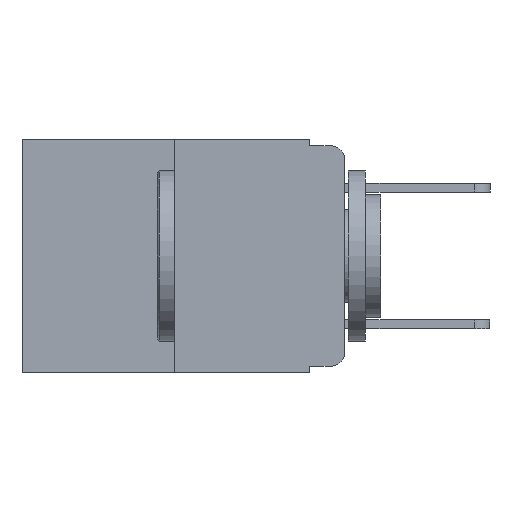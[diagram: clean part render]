
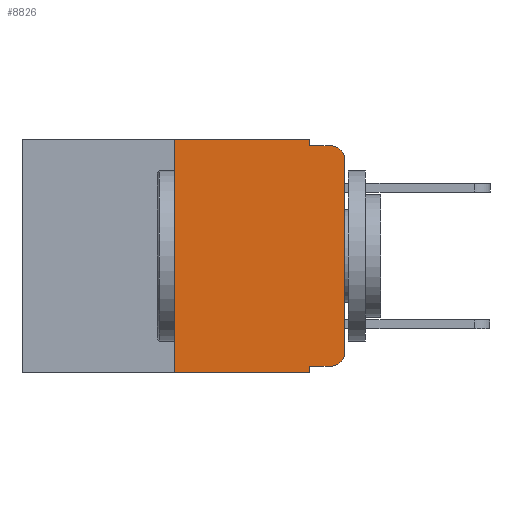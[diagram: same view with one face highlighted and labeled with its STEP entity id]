
A CAD part, left-side view. The second image highlights one B-rep face of the part: STEP entity #8826.
In plain terms, the highlighted planar face has unit normal (-1, 0, 0).
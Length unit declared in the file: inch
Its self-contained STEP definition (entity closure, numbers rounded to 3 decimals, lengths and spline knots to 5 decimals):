
#76 = ORIENTED_EDGE ( 'NONE', *, *, #11005, .F. ) ;
#257 = EDGE_CURVE ( 'NONE', #10354, #1888, #15222, .T. ) ;
#269 = DIRECTION ( 'NONE',  ( 1., 0., 0. ) ) ;
#712 = AXIS2_PLACEMENT_3D ( 'NONE', #13925, #269, #10155 ) ;
#747 = LINE ( 'NONE', #17176, #7976 ) ;
#757 = CARTESIAN_POINT ( 'NONE',  ( 0., 0., -0.313 ) ) ;
#927 = VECTOR ( 'NONE', #12690, 39.37008 ) ;
#973 = VECTOR ( 'NONE', #11604, 39.37008 ) ;
#1206 = EDGE_CURVE ( 'NONE', #1888, #14807, #6623, .T. ) ;
#1469 = LINE ( 'NONE', #15283, #973 ) ;
#1518 = CARTESIAN_POINT ( 'NONE',  ( 0., 0.02, -0.01 ) ) ;
#1888 = VERTEX_POINT ( 'NONE', #11356 ) ;
#2137 = ORIENTED_EDGE ( 'NONE', *, *, #10632, .T. ) ;
#2163 = VECTOR ( 'NONE', #12862, 39.37008 ) ;
#2236 = EDGE_CURVE ( 'NONE', #11568, #10518, #9828, .T. ) ;
#2255 = EDGE_CURVE ( 'NONE', #17080, #9386, #5489, .T. ) ;
#2849 = DIRECTION ( 'NONE',  ( 0., -1., 0. ) ) ;
#3231 = CARTESIAN_POINT ( 'NONE',  ( 0., 0.051, -0.01 ) ) ;
#3321 = EDGE_CURVE ( 'NONE', #9386, #14807, #747, .T. ) ;
#3377 = PLANE ( 'NONE',  #712 ) ;
#3737 = DIRECTION ( 'NONE',  ( 0., -1., 0. ) ) ;
#4075 = ORIENTED_EDGE ( 'NONE', *, *, #2236, .F. ) ;
#4689 = EDGE_CURVE ( 'NONE', #10503, #7376, #1469, .T. ) ;
#4737 = EDGE_CURVE ( 'NONE', #11568, #14059, #14131, .T. ) ;
#5237 = ORIENTED_EDGE ( 'NONE', *, *, #3321, .F. ) ;
#5489 = LINE ( 'NONE', #14955, #8638 ) ;
#5606 = CARTESIAN_POINT ( 'NONE',  ( 0., 0.02, -0.313 ) ) ;
#5688 = AXIS2_PLACEMENT_3D ( 'NONE', #5606, #14610, #6977 ) ;
#6395 = CARTESIAN_POINT ( 'NONE',  ( 0., 0.473, 0. ) ) ;
#6471 = CARTESIAN_POINT ( 'NONE',  ( 0., 0.051, -0.333 ) ) ;
#6623 = CIRCLE ( 'NONE', #15960, 0.02 ) ;
#6977 = DIRECTION ( 'NONE',  ( 0., 0., -1. ) ) ;
#7217 = DIRECTION ( 'NONE',  ( 0., 0., -1. ) ) ;
#7234 = EDGE_CURVE ( 'NONE', #14059, #10354, #10502, .T. ) ;
#7376 = VERTEX_POINT ( 'NONE', #16024 ) ;
#7976 = VECTOR ( 'NONE', #15986, 39.37008 ) ;
#8301 = CARTESIAN_POINT ( 'NONE',  ( 0., 0.051, -0.333 ) ) ;
#8638 = VECTOR ( 'NONE', #12142, 39.37008 ) ;
#8648 = ORIENTED_EDGE ( 'NONE', *, *, #2255, .F. ) ;
#8799 = ORIENTED_EDGE ( 'NONE', *, *, #1206, .T. ) ;
#8826 = ADVANCED_FACE ( 'NONE', ( #9641 ), #3377, .F. ) ;
#9386 = VERTEX_POINT ( 'NONE', #3231 ) ;
#9641 = FACE_OUTER_BOUND ( 'NONE', #16081, .T. ) ;
#9761 = CARTESIAN_POINT ( 'NONE',  ( 0., 0.02, -0.333 ) ) ;
#9828 = LINE ( 'NONE', #13721, #16071 ) ;
#10155 = DIRECTION ( 'NONE',  ( 0., 0., -1. ) ) ;
#10354 = VERTEX_POINT ( 'NONE', #757 ) ;
#10502 = CIRCLE ( 'NONE', #5688, 0.02 ) ;
#10503 = VERTEX_POINT ( 'NONE', #10765 ) ;
#10518 = VERTEX_POINT ( 'NONE', #15760 ) ;
#10632 = EDGE_CURVE ( 'NONE', #10503, #10518, #16743, .T. ) ;
#10765 = CARTESIAN_POINT ( 'NONE',  ( 0., 0.25, -0.343 ) ) ;
#10786 = VECTOR ( 'NONE', #3737, 39.37008 ) ;
#11005 = EDGE_CURVE ( 'NONE', #7376, #17080, #16560, .T. ) ;
#11145 = DIRECTION ( 'NONE',  ( 0., 0., -1. ) ) ;
#11356 = CARTESIAN_POINT ( 'NONE',  ( 0., 0., -0.03 ) ) ;
#11500 = CARTESIAN_POINT ( 'NONE',  ( 0., 0.051, 0. ) ) ;
#11568 = VERTEX_POINT ( 'NONE', #8301 ) ;
#11604 = DIRECTION ( 'NONE',  ( 0., 0., 1. ) ) ;
#12142 = DIRECTION ( 'NONE',  ( 0., 0., -1. ) ) ;
#12284 = CARTESIAN_POINT ( 'NONE',  ( 0., 0.473, -0.343 ) ) ;
#12690 = DIRECTION ( 'NONE',  ( 0., 0., 1. ) ) ;
#12862 = DIRECTION ( 'NONE',  ( 0., -1., 0. ) ) ;
#13561 = ORIENTED_EDGE ( 'NONE', *, *, #4737, .T. ) ;
#13712 = ORIENTED_EDGE ( 'NONE', *, *, #257, .T. ) ;
#13721 = CARTESIAN_POINT ( 'NONE',  ( 0., 0.051, 0. ) ) ;
#13925 = CARTESIAN_POINT ( 'NONE',  ( 0., 0.473, 0. ) ) ;
#14059 = VERTEX_POINT ( 'NONE', #9761 ) ;
#14131 = LINE ( 'NONE', #6471, #10786 ) ;
#14610 = DIRECTION ( 'NONE',  ( -1., 0., 0. ) ) ;
#14689 = VECTOR ( 'NONE', #2849, 39.37008 ) ;
#14745 = CARTESIAN_POINT ( 'NONE',  ( 0., 0., 0. ) ) ;
#14807 = VERTEX_POINT ( 'NONE', #1518 ) ;
#14955 = CARTESIAN_POINT ( 'NONE',  ( 0., 0.051, 0. ) ) ;
#15222 = LINE ( 'NONE', #14745, #927 ) ;
#15271 = ORIENTED_EDGE ( 'NONE', *, *, #7234, .T. ) ;
#15283 = CARTESIAN_POINT ( 'NONE',  ( 0., 0.25, 0. ) ) ;
#15324 = DIRECTION ( 'NONE',  ( -1., 0., 0. ) ) ;
#15531 = CARTESIAN_POINT ( 'NONE',  ( 0., 0.02, -0.03 ) ) ;
#15760 = CARTESIAN_POINT ( 'NONE',  ( 0., 0.051, -0.343 ) ) ;
#15960 = AXIS2_PLACEMENT_3D ( 'NONE', #15531, #15324, #11145 ) ;
#15986 = DIRECTION ( 'NONE',  ( 0., -1., 0. ) ) ;
#16024 = CARTESIAN_POINT ( 'NONE',  ( 0., 0.25, 0. ) ) ;
#16071 = VECTOR ( 'NONE', #7217, 39.37008 ) ;
#16081 = EDGE_LOOP ( 'NONE', ( #13712, #8799, #5237, #8648, #76, #17030, #2137, #4075, #13561, #15271 ) ) ;
#16560 = LINE ( 'NONE', #6395, #2163 ) ;
#16743 = LINE ( 'NONE', #12284, #14689 ) ;
#17030 = ORIENTED_EDGE ( 'NONE', *, *, #4689, .F. ) ;
#17080 = VERTEX_POINT ( 'NONE', #11500 ) ;
#17176 = CARTESIAN_POINT ( 'NONE',  ( 0., 0.051, -0.01 ) ) ;
